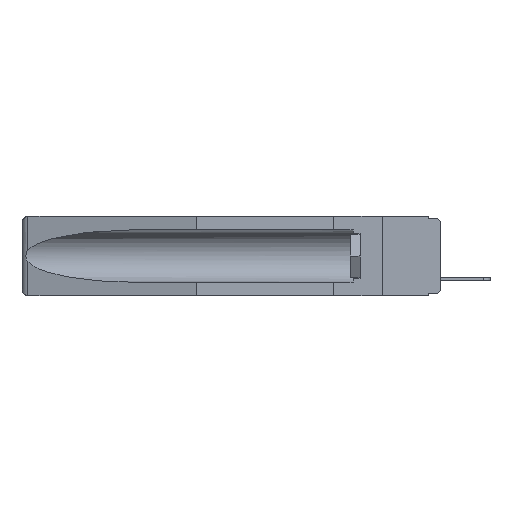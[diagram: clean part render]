
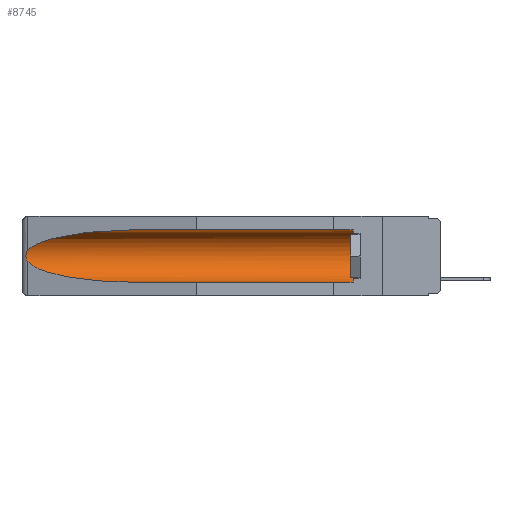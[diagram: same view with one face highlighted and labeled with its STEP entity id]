
A CAD part, left-side view. The second image highlights one B-rep face of the part: STEP entity #8745.
In plain terms, the highlighted cylindrical face has radius 2.857 mm (diameter 5.715 mm), a partial arc.
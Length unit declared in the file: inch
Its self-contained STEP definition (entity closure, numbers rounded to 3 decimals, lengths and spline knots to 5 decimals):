
#507 = EDGE_CURVE ( 'NONE', #1865, #589, #9554, .T. ) ;
#589 = VERTEX_POINT ( 'NONE', #10790 ) ;
#1142 = CARTESIAN_POINT ( 'NONE',  ( 0.21114, 1.30732, -0.284 ) ) ;
#1865 = VERTEX_POINT ( 'NONE', #10108 ) ;
#1874 = CARTESIAN_POINT ( 'NONE',  ( 0.26597, 1.52961, -0.15275 ) ) ;
#2240 = ORIENTED_EDGE ( 'NONE', *, *, #6121, .T. ) ;
#2656 = CARTESIAN_POINT ( 'NONE',  ( 0.25451, 1.48313, -0.09465 ) ) ;
#3087 = CARTESIAN_POINT ( 'NONE',  ( 0.155, -0.30754, -0.059 ) ) ;
#3244 = CARTESIAN_POINT ( 'NONE',  ( 0.2673, 1.5327, -0.16383 ) ) ;
#3428 = CARTESIAN_POINT ( 'NONE',  ( 0.26654, 1.53092, -0.15636 ) ) ;
#3786 = CARTESIAN_POINT ( 'NONE',  ( 0.155, 0.126, -0.059 ) ) ;
#3991 = CARTESIAN_POINT ( 'NONE',  ( 0.155, 1.07973, -0.284 ) ) ;
#4018 = EDGE_CURVE ( 'NONE', #10777, #10096, #9430, .T. ) ;
#4367 = EDGE_CURVE ( 'NONE', #10096, #1865, #14138, .T. ) ;
#5395 = CARTESIAN_POINT ( 'NONE',  ( 0.26537, 1.52718, -0.14972 ) ) ;
#5598 = VERTEX_POINT ( 'NONE', #17985 ) ;
#5796 = CYLINDRICAL_SURFACE ( 'NONE', #16105, 0.1125 ) ;
#6121 = EDGE_CURVE ( 'NONE', #589, #5598, #9900, .T. ) ;
#6232 = CARTESIAN_POINT ( 'NONE',  ( 0.26655, 1.53094, -0.18657 ) ) ;
#6251 = DIRECTION ( 'NONE',  ( 0., -1., 0. ) ) ;
#6424 = CARTESIAN_POINT ( 'NONE',  ( 0.155, 0.126, -0.1715 ) ) ;
#6443 = CIRCLE ( 'NONE', #14953, 0.1125 ) ;
#7512 = CARTESIAN_POINT ( 'NONE',  ( 0.2675, 1.53308, -0.17534 ) ) ;
#7812 = DIRECTION ( 'NONE',  ( 0., 1., 0. ) ) ;
#8330 = CARTESIAN_POINT ( 'NONE',  ( 0.155, 0.126, -0.284 ) ) ;
#8676 = EDGE_CURVE ( 'NONE', #13164, #10777, #6443, .T. ) ;
#8745 = ADVANCED_FACE ( 'NONE', ( #8814 ), #5796, .F. ) ;
#8814 = FACE_OUTER_BOUND ( 'NONE', #16178, .T. ) ;
#8883 = CARTESIAN_POINT ( 'NONE',  ( 0.26537, 1.52718, -0.19328 ) ) ;
#9430 = LINE ( 'NONE', #3087, #17281 ) ;
#9554 = B_SPLINE_CURVE_WITH_KNOTS ( 'NONE', 3,
 ( #15895, #1874, #3428, #3244, #14539, #7512, #17222, #6232, #11685, #8883 ),
 .UNSPECIFIED., .F., .F.,
 ( 4, 2, 2, 2, 4 ),
 ( 0., 0.00029, 0.00058, 0.00087, 0.00117 ),
 .UNSPECIFIED. ) ;
#9900 =( BOUNDED_CURVE ( )  B_SPLINE_CURVE ( 3, ( #15976, #17831, #1142, #3991 ),
 .UNSPECIFIED., .F., .F. ) 
 B_SPLINE_CURVE_WITH_KNOTS ( ( 4, 4 ),
 ( 0.1948, 1.5708 ),
 .UNSPECIFIED. ) 
 CURVE ( )  GEOMETRIC_REPRESENTATION_ITEM ( )  RATIONAL_B_SPLINE_CURVE ( ( 1., 0.848, 0.848, 1. ) ) 
 REPRESENTATION_ITEM ( '' )  );
#10096 = VERTEX_POINT ( 'NONE', #10822 ) ;
#10108 = CARTESIAN_POINT ( 'NONE',  ( 0.26537, 1.52718, -0.14972 ) ) ;
#10389 = VECTOR ( 'NONE', #14715, 39.37008 ) ;
#10472 = CARTESIAN_POINT ( 'NONE',  ( 0.155, 1.07973, -0.059 ) ) ;
#10777 = VERTEX_POINT ( 'NONE', #3786 ) ;
#10790 = CARTESIAN_POINT ( 'NONE',  ( 0.26537, 1.52718, -0.19328 ) ) ;
#10822 = CARTESIAN_POINT ( 'NONE',  ( 0.155, 1.07973, -0.059 ) ) ;
#11599 = ORIENTED_EDGE ( 'NONE', *, *, #8676, .T. ) ;
#11616 = ORIENTED_EDGE ( 'NONE', *, *, #16346, .F. ) ;
#11659 = ORIENTED_EDGE ( 'NONE', *, *, #4367, .T. ) ;
#11685 = CARTESIAN_POINT ( 'NONE',  ( 0.26597, 1.5296, -0.19026 ) ) ;
#11894 = CARTESIAN_POINT ( 'NONE',  ( 0.21114, 1.30732, -0.059 ) ) ;
#11917 = CARTESIAN_POINT ( 'NONE',  ( 0.155, -0.30754, -0.284 ) ) ;
#12323 = ORIENTED_EDGE ( 'NONE', *, *, #507, .T. ) ;
#12751 = DIRECTION ( 'NONE',  ( 0., 1., 0. ) ) ;
#13164 = VERTEX_POINT ( 'NONE', #8330 ) ;
#13406 = CARTESIAN_POINT ( 'NONE',  ( 0.155, -0.30754, -0.1715 ) ) ;
#14138 =( BOUNDED_CURVE ( )  B_SPLINE_CURVE ( 3, ( #10472, #11894, #2656, #5395 ),
 .UNSPECIFIED., .F., .F. ) 
 B_SPLINE_CURVE_WITH_KNOTS ( ( 4, 4 ),
 ( 4.71239, 6.08839 ),
 .UNSPECIFIED. ) 
 CURVE ( )  GEOMETRIC_REPRESENTATION_ITEM ( )  RATIONAL_B_SPLINE_CURVE ( ( 1., 0.848, 0.848, 1. ) ) 
 REPRESENTATION_ITEM ( '' )  );
#14539 = CARTESIAN_POINT ( 'NONE',  ( 0.2675, 1.53308, -0.16763 ) ) ;
#14627 = DIRECTION ( 'NONE',  ( 0., 0., 1. ) ) ;
#14715 = DIRECTION ( 'NONE',  ( 0., 1., 0. ) ) ;
#14953 = AXIS2_PLACEMENT_3D ( 'NONE', #6424, #6251, #14627 ) ;
#15630 = LINE ( 'NONE', #11917, #10389 ) ;
#15895 = CARTESIAN_POINT ( 'NONE',  ( 0.26537, 1.52718, -0.14972 ) ) ;
#15976 = CARTESIAN_POINT ( 'NONE',  ( 0.26537, 1.52718, -0.19328 ) ) ;
#16105 = AXIS2_PLACEMENT_3D ( 'NONE', #13406, #7812, #17364 ) ;
#16178 = EDGE_LOOP ( 'NONE', ( #11659, #12323, #2240, #11616, #11599, #17327 ) ) ;
#16346 = EDGE_CURVE ( 'NONE', #13164, #5598, #15630, .T. ) ;
#17222 = CARTESIAN_POINT ( 'NONE',  ( 0.2673, 1.53269, -0.17917 ) ) ;
#17281 = VECTOR ( 'NONE', #12751, 39.37008 ) ;
#17327 = ORIENTED_EDGE ( 'NONE', *, *, #4018, .T. ) ;
#17364 = DIRECTION ( 'NONE',  ( 0., 0., 1. ) ) ;
#17831 = CARTESIAN_POINT ( 'NONE',  ( 0.25451, 1.48313, -0.24835 ) ) ;
#17985 = CARTESIAN_POINT ( 'NONE',  ( 0.155, 1.07973, -0.284 ) ) ;
